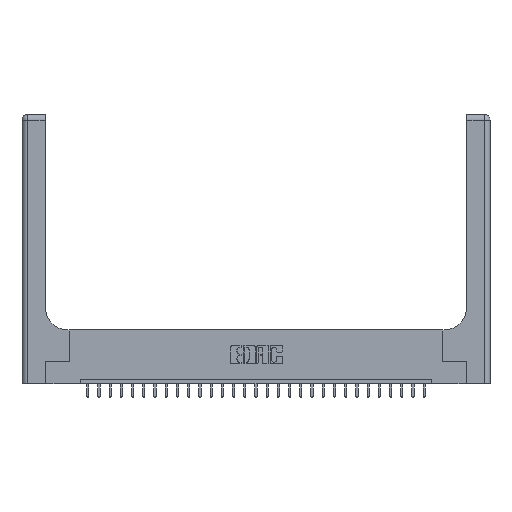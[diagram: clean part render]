
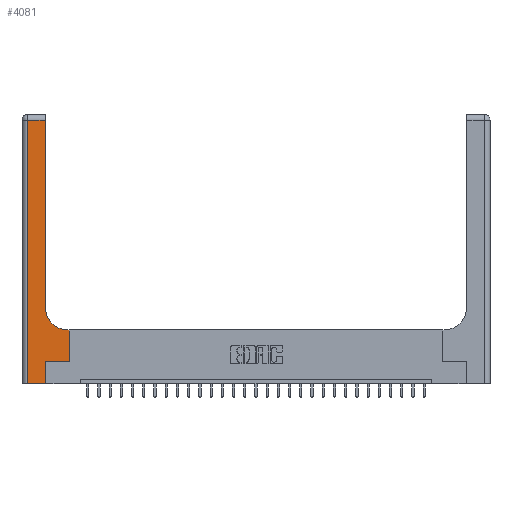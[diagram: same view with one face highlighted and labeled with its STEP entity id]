
A CAD part, top view. The second image highlights one B-rep face of the part: STEP entity #4081.
In plain terms, the highlighted planar face has unit normal (0, 0, 1).
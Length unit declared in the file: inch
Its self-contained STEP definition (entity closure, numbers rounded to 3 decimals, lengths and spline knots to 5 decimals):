
#99 = CARTESIAN_POINT ( 'NONE',  ( 0.265, 0.25, 0.37 ) ) ;
#206 = CARTESIAN_POINT ( 'NONE',  ( 0.26, 0.6, 0.37 ) ) ;
#717 = VERTEX_POINT ( 'NONE', #17181 ) ;
#806 = CARTESIAN_POINT ( 'NONE',  ( 0.51, 0.85, 0.37 ) ) ;
#905 = DIRECTION ( 'NONE',  ( 0., 1., 0. ) ) ;
#1643 = VERTEX_POINT ( 'NONE', #21759 ) ;
#2198 = DIRECTION ( 'NONE',  ( 1., 0., 0. ) ) ;
#2243 = DIRECTION ( 'NONE',  ( -1., 0., 0. ) ) ;
#2258 = LINE ( 'NONE', #18259, #3130 ) ;
#2564 = EDGE_CURVE ( 'NONE', #18988, #15446, #13144, .T. ) ;
#2826 = VECTOR ( 'NONE', #6344, 39.37008 ) ;
#3080 = VECTOR ( 'NONE', #6714, 39.37008 ) ;
#3090 = EDGE_CURVE ( 'NONE', #24994, #12077, #13940, .T. ) ;
#3130 = VECTOR ( 'NONE', #22006, 39.37008 ) ;
#3625 = EDGE_CURVE ( 'NONE', #19717, #18988, #5323, .T. ) ;
#4081 = ADVANCED_FACE ( 'NONE', ( #12424 ), #14806, .F. ) ;
#4169 = ORIENTED_EDGE ( 'NONE', *, *, #4875, .T. ) ;
#4480 = CARTESIAN_POINT ( 'NONE',  ( 0.26, 3., 0.37 ) ) ;
#4648 = VECTOR ( 'NONE', #25739, 39.37008 ) ;
#4875 = EDGE_CURVE ( 'NONE', #717, #1643, #16226, .T. ) ;
#5019 = AXIS2_PLACEMENT_3D ( 'NONE', #806, #24814, #6789 ) ;
#5323 = LINE ( 'NONE', #9454, #4648 ) ;
#6323 = CARTESIAN_POINT ( 'NONE',  ( 0., 0., 0.37 ) ) ;
#6336 = VECTOR ( 'NONE', #17334, 39.37008 ) ;
#6344 = DIRECTION ( 'NONE',  ( 0., 1., 0. ) ) ;
#6702 = DIRECTION ( 'NONE',  ( 0., 0., -1. ) ) ;
#6714 = DIRECTION ( 'NONE',  ( -1., 0., 0. ) ) ;
#6728 = CARTESIAN_POINT ( 'NONE',  ( 0.528, 0.6, 0.37 ) ) ;
#6789 = DIRECTION ( 'NONE',  ( 1., 0., 0. ) ) ;
#6925 = ORIENTED_EDGE ( 'NONE', *, *, #21629, .T. ) ;
#7197 = CARTESIAN_POINT ( 'NONE',  ( 0.265, 0., 0.37 ) ) ;
#8117 = ORIENTED_EDGE ( 'NONE', *, *, #3625, .T. ) ;
#8237 = VERTEX_POINT ( 'NONE', #10212 ) ;
#8255 = CARTESIAN_POINT ( 'NONE',  ( 0.528, 0.25, 0.37 ) ) ;
#9145 = CARTESIAN_POINT ( 'NONE',  ( 0.528, 0.25, 0.37 ) ) ;
#9454 = CARTESIAN_POINT ( 'NONE',  ( 0.265, 0.25, 0.37 ) ) ;
#9656 = ORIENTED_EDGE ( 'NONE', *, *, #20843, .T. ) ;
#9764 = ORIENTED_EDGE ( 'NONE', *, *, #18443, .T. ) ;
#10039 = EDGE_LOOP ( 'NONE', ( #9764, #4169, #25152, #15905, #9656, #8117, #22365, #6925, #16235 ) ) ;
#10125 = CARTESIAN_POINT ( 'NONE',  ( 0.26, 0.85, 0.37 ) ) ;
#10212 = CARTESIAN_POINT ( 'NONE',  ( 0.265, 0., 0.37 ) ) ;
#10236 = VECTOR ( 'NONE', #2243, 39.37008 ) ;
#12077 = VERTEX_POINT ( 'NONE', #10125 ) ;
#12082 = CARTESIAN_POINT ( 'NONE',  ( 0.51, 0.6, 0.37 ) ) ;
#12424 = FACE_OUTER_BOUND ( 'NONE', #10039, .T. ) ;
#12827 = LINE ( 'NONE', #206, #3080 ) ;
#13144 = LINE ( 'NONE', #9145, #22816 ) ;
#13774 = VECTOR ( 'NONE', #2198, 39.37008 ) ;
#13940 = CIRCLE ( 'NONE', #5019, 0.25 ) ;
#14806 = PLANE ( 'NONE',  #26362 ) ;
#15446 = VERTEX_POINT ( 'NONE', #6728 ) ;
#15905 = ORIENTED_EDGE ( 'NONE', *, *, #23689, .T. ) ;
#16226 = LINE ( 'NONE', #20254, #10236 ) ;
#16235 = ORIENTED_EDGE ( 'NONE', *, *, #3090, .T. ) ;
#17181 = CARTESIAN_POINT ( 'NONE',  ( 0.26, 2.94, 0.37 ) ) ;
#17334 = DIRECTION ( 'NONE',  ( 0., 1., 0. ) ) ;
#18259 = CARTESIAN_POINT ( 'NONE',  ( 0.06, 3., 0.37 ) ) ;
#18443 = EDGE_CURVE ( 'NONE', #12077, #717, #24627, .T. ) ;
#18453 = CARTESIAN_POINT ( 'NONE',  ( 0.06, 0., 0.37 ) ) ;
#18988 = VERTEX_POINT ( 'NONE', #8255 ) ;
#19210 = LINE ( 'NONE', #7197, #6336 ) ;
#19717 = VERTEX_POINT ( 'NONE', #99 ) ;
#20254 = CARTESIAN_POINT ( 'NONE',  ( 0., 2.94, 0.37 ) ) ;
#20278 = VERTEX_POINT ( 'NONE', #18453 ) ;
#20580 = DIRECTION ( 'NONE',  ( -1., 0., 0. ) ) ;
#20598 = LINE ( 'NONE', #6323, #13774 ) ;
#20843 = EDGE_CURVE ( 'NONE', #8237, #19717, #19210, .T. ) ;
#20975 = CARTESIAN_POINT ( 'NONE',  ( 0., 3., 0.37 ) ) ;
#21629 = EDGE_CURVE ( 'NONE', #15446, #24994, #12827, .T. ) ;
#21759 = CARTESIAN_POINT ( 'NONE',  ( 0.06, 2.94, 0.37 ) ) ;
#22006 = DIRECTION ( 'NONE',  ( 0., -1., 0. ) ) ;
#22365 = ORIENTED_EDGE ( 'NONE', *, *, #2564, .T. ) ;
#22816 = VECTOR ( 'NONE', #905, 39.37008 ) ;
#23360 = EDGE_CURVE ( 'NONE', #1643, #20278, #2258, .T. ) ;
#23689 = EDGE_CURVE ( 'NONE', #20278, #8237, #20598, .T. ) ;
#24627 = LINE ( 'NONE', #4480, #2826 ) ;
#24814 = DIRECTION ( 'NONE',  ( 0., 0., -1. ) ) ;
#24994 = VERTEX_POINT ( 'NONE', #12082 ) ;
#25152 = ORIENTED_EDGE ( 'NONE', *, *, #23360, .T. ) ;
#25739 = DIRECTION ( 'NONE',  ( 1., 0., 0. ) ) ;
#26362 = AXIS2_PLACEMENT_3D ( 'NONE', #20975, #6702, #20580 ) ;
